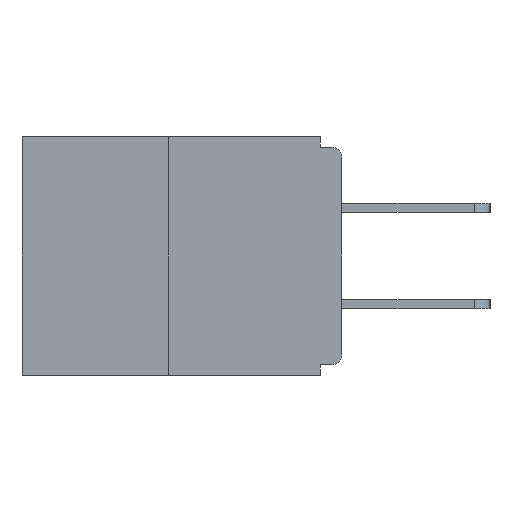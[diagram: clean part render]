
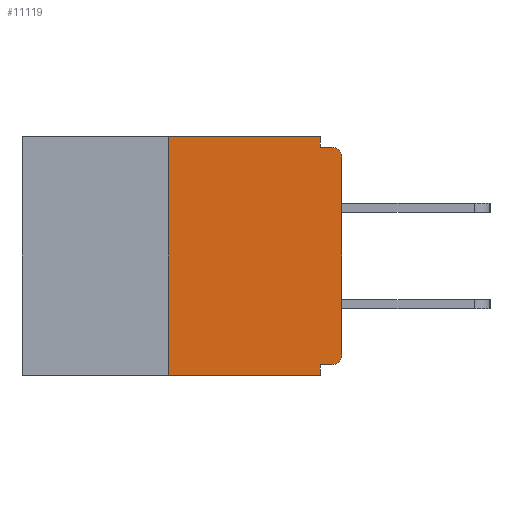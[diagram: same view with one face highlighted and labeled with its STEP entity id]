
A CAD part, left-side view. The second image highlights one B-rep face of the part: STEP entity #11119.
In plain terms, the highlighted planar face has unit normal (-1, 0, 0).
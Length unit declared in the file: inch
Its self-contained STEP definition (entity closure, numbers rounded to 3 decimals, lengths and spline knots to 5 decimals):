
#130 = CARTESIAN_POINT ( 'NONE',  ( 0., 0.015, -0.03 ) ) ;
#212 = LINE ( 'NONE', #636, #9962 ) ;
#260 = LINE ( 'NONE', #1173, #9638 ) ;
#636 = CARTESIAN_POINT ( 'NONE',  ( 0., 0., 0. ) ) ;
#1016 = ORIENTED_EDGE ( 'NONE', *, *, #5339, .T. ) ;
#1173 = CARTESIAN_POINT ( 'NONE',  ( 0., 0., -0.328 ) ) ;
#1311 = AXIS2_PLACEMENT_3D ( 'NONE', #9770, #4856, #7431 ) ;
#1511 = ORIENTED_EDGE ( 'NONE', *, *, #12914, .T. ) ;
#1633 = VERTEX_POINT ( 'NONE', #5884 ) ;
#1722 = CARTESIAN_POINT ( 'NONE',  ( 0., 0.015, -0.328 ) ) ;
#2080 = EDGE_CURVE ( 'NONE', #15730, #5757, #3386, .T. ) ;
#2436 = VECTOR ( 'NONE', #14212, 39.37008 ) ;
#2581 = DIRECTION ( 'NONE',  ( -1., 0., 0. ) ) ;
#2672 = CARTESIAN_POINT ( 'NONE',  ( 0., 0.031, -0.343 ) ) ;
#2683 = ORIENTED_EDGE ( 'NONE', *, *, #11128, .T. ) ;
#2687 = CARTESIAN_POINT ( 'NONE',  ( 0., 0.031, -0.343 ) ) ;
#3030 = CARTESIAN_POINT ( 'NONE',  ( 0., 0.46, 0. ) ) ;
#3205 = CARTESIAN_POINT ( 'NONE',  ( 0., 0.46, 0. ) ) ;
#3386 = LINE ( 'NONE', #3030, #10118 ) ;
#3439 = VERTEX_POINT ( 'NONE', #10125 ) ;
#3898 = ORIENTED_EDGE ( 'NONE', *, *, #11584, .F. ) ;
#4066 = ORIENTED_EDGE ( 'NONE', *, *, #10182, .F. ) ;
#4259 = VECTOR ( 'NONE', #11493, 39.37008 ) ;
#4805 = VERTEX_POINT ( 'NONE', #9059 ) ;
#4856 = DIRECTION ( 'NONE',  ( -1., 0., 0. ) ) ;
#4940 = DIRECTION ( 'NONE',  ( 0., 0., -1. ) ) ;
#5339 = EDGE_CURVE ( 'NONE', #12662, #6732, #13871, .T. ) ;
#5376 = VERTEX_POINT ( 'NONE', #6064 ) ;
#5568 = VECTOR ( 'NONE', #11334, 39.37008 ) ;
#5757 = VERTEX_POINT ( 'NONE', #9210 ) ;
#5884 = CARTESIAN_POINT ( 'NONE',  ( 0., 0., -0.03 ) ) ;
#6064 = CARTESIAN_POINT ( 'NONE',  ( 0., 0.031, -0.328 ) ) ;
#6173 = DIRECTION ( 'NONE',  ( 0., -1., 0. ) ) ;
#6414 = DIRECTION ( 'NONE',  ( 0., 0., -1. ) ) ;
#6423 = LINE ( 'NONE', #2672, #7688 ) ;
#6513 = DIRECTION ( 'NONE',  ( 0., -1., 0. ) ) ;
#6705 = DIRECTION ( 'NONE',  ( 0., 0., 1. ) ) ;
#6732 = VERTEX_POINT ( 'NONE', #8165 ) ;
#7227 = LINE ( 'NONE', #8185, #2436 ) ;
#7233 = DIRECTION ( 'NONE',  ( 1., 0., 0. ) ) ;
#7431 = DIRECTION ( 'NONE',  ( 0., 0., -1. ) ) ;
#7688 = VECTOR ( 'NONE', #6414, 39.37008 ) ;
#8165 = CARTESIAN_POINT ( 'NONE',  ( 0., 0., -0.313 ) ) ;
#8185 = CARTESIAN_POINT ( 'NONE',  ( 0., 0.031, 0. ) ) ;
#8632 = DIRECTION ( 'NONE',  ( 0., 0., -1. ) ) ;
#8856 = LINE ( 'NONE', #9635, #5568 ) ;
#8908 = ORIENTED_EDGE ( 'NONE', *, *, #13787, .F. ) ;
#9059 = CARTESIAN_POINT ( 'NONE',  ( 0., 0.25, -0.343 ) ) ;
#9192 = ORIENTED_EDGE ( 'NONE', *, *, #14085, .F. ) ;
#9210 = CARTESIAN_POINT ( 'NONE',  ( 0., 0.031, 0. ) ) ;
#9635 = CARTESIAN_POINT ( 'NONE',  ( 0., 0.46, -0.343 ) ) ;
#9638 = VECTOR ( 'NONE', #14627, 39.37008 ) ;
#9770 = CARTESIAN_POINT ( 'NONE',  ( 0., 0.015, -0.313 ) ) ;
#9962 = VECTOR ( 'NONE', #6705, 39.37008 ) ;
#10118 = VECTOR ( 'NONE', #6513, 39.37008 ) ;
#10125 = CARTESIAN_POINT ( 'NONE',  ( 0., 0.031, -0.015 ) ) ;
#10182 = EDGE_CURVE ( 'NONE', #4805, #15730, #12897, .T. ) ;
#10569 = CARTESIAN_POINT ( 'NONE',  ( 0., 0.25, 0. ) ) ;
#10570 = PLANE ( 'NONE',  #15487 ) ;
#10970 = VERTEX_POINT ( 'NONE', #2687 ) ;
#11119 = ADVANCED_FACE ( 'NONE', ( #11719 ), #10570, .F. ) ;
#11122 = ORIENTED_EDGE ( 'NONE', *, *, #2080, .F. ) ;
#11128 = EDGE_CURVE ( 'NONE', #4805, #10970, #8856, .T. ) ;
#11334 = DIRECTION ( 'NONE',  ( 0., -1., 0. ) ) ;
#11384 = EDGE_CURVE ( 'NONE', #1633, #12507, #12480, .T. ) ;
#11493 = DIRECTION ( 'NONE',  ( 0., 0., 1. ) ) ;
#11504 = LINE ( 'NONE', #13629, #14379 ) ;
#11584 = EDGE_CURVE ( 'NONE', #12662, #5376, #260, .T. ) ;
#11588 = ORIENTED_EDGE ( 'NONE', *, *, #11384, .T. ) ;
#11702 = EDGE_CURVE ( 'NONE', #3439, #12507, #11504, .T. ) ;
#11719 = FACE_OUTER_BOUND ( 'NONE', #12512, .T. ) ;
#12356 = CARTESIAN_POINT ( 'NONE',  ( 0., 0.25, 0. ) ) ;
#12480 = CIRCLE ( 'NONE', #15790, 0.015 ) ;
#12507 = VERTEX_POINT ( 'NONE', #14203 ) ;
#12512 = EDGE_LOOP ( 'NONE', ( #11122, #4066, #2683, #9192, #3898, #1016, #1511, #11588, #14425, #8908 ) ) ;
#12662 = VERTEX_POINT ( 'NONE', #1722 ) ;
#12897 = LINE ( 'NONE', #10569, #4259 ) ;
#12914 = EDGE_CURVE ( 'NONE', #6732, #1633, #212, .T. ) ;
#13629 = CARTESIAN_POINT ( 'NONE',  ( 0., 0., -0.015 ) ) ;
#13787 = EDGE_CURVE ( 'NONE', #5757, #3439, #7227, .T. ) ;
#13871 = CIRCLE ( 'NONE', #1311, 0.015 ) ;
#14085 = EDGE_CURVE ( 'NONE', #5376, #10970, #6423, .T. ) ;
#14203 = CARTESIAN_POINT ( 'NONE',  ( 0., 0.015, -0.015 ) ) ;
#14212 = DIRECTION ( 'NONE',  ( 0., 0., -1. ) ) ;
#14379 = VECTOR ( 'NONE', #6173, 39.37008 ) ;
#14425 = ORIENTED_EDGE ( 'NONE', *, *, #11702, .F. ) ;
#14627 = DIRECTION ( 'NONE',  ( 0., 1., 0. ) ) ;
#15487 = AXIS2_PLACEMENT_3D ( 'NONE', #3205, #7233, #8632 ) ;
#15730 = VERTEX_POINT ( 'NONE', #12356 ) ;
#15790 = AXIS2_PLACEMENT_3D ( 'NONE', #130, #2581, #4940 ) ;
